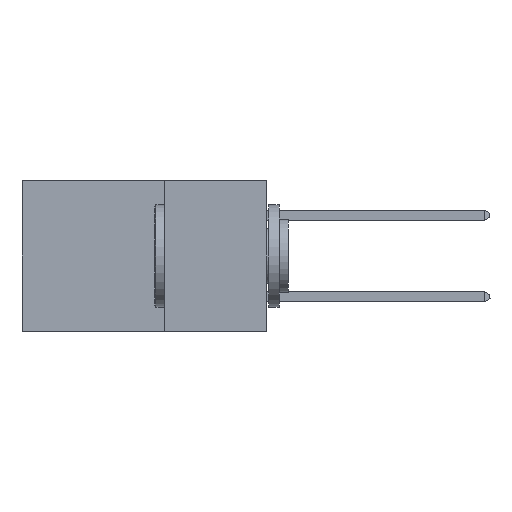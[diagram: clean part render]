
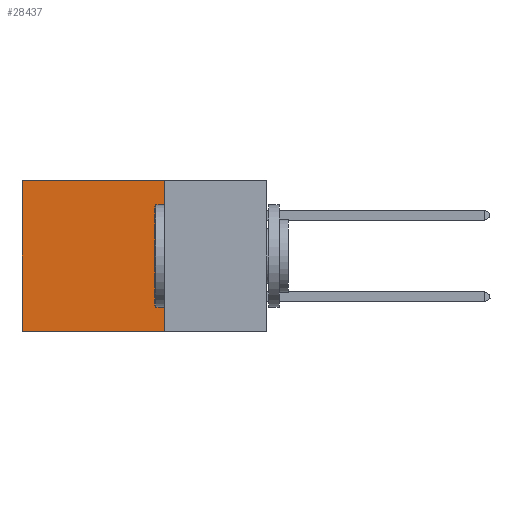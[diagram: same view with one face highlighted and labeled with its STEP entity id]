
A CAD part, left-side view. The second image highlights one B-rep face of the part: STEP entity #28437.
In plain terms, the highlighted planar face has unit normal (-1, 0, 0).
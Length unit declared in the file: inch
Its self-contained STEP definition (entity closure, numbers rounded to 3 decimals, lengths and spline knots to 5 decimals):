
#145 = CARTESIAN_POINT ( 'NONE',  ( 0.2875, 0.25, 0. ) ) ;
#192 = DIRECTION ( 'NONE',  ( 0., 1., 0. ) ) ;
#413 = CARTESIAN_POINT ( 'NONE',  ( 0.2875, 0.25, -0.37 ) ) ;
#705 = VERTEX_POINT ( 'NONE', #12265 ) ;
#2014 = VECTOR ( 'NONE', #17488, 39.37008 ) ;
#2131 = EDGE_CURVE ( 'NONE', #24202, #2950, #23606, .T. ) ;
#2950 = VERTEX_POINT ( 'NONE', #413 ) ;
#4762 = CARTESIAN_POINT ( 'NONE',  ( 0.2875, 0.25, -0.37 ) ) ;
#5652 = VECTOR ( 'NONE', #17753, 39.37008 ) ;
#5959 = EDGE_LOOP ( 'NONE', ( #19941, #28131, #9766, #14712 ) ) ;
#6461 = CARTESIAN_POINT ( 'NONE',  ( 0.2875, 0.6, -0.37 ) ) ;
#6471 = CARTESIAN_POINT ( 'NONE',  ( 0.2875, 0.25, 0. ) ) ;
#7491 = DIRECTION ( 'NONE',  ( 1., 0., 0. ) ) ;
#9766 = ORIENTED_EDGE ( 'NONE', *, *, #2131, .F. ) ;
#10744 = CARTESIAN_POINT ( 'NONE',  ( 0.2875, 0.6, 0. ) ) ;
#11855 = CARTESIAN_POINT ( 'NONE',  ( 0.2875, 0.25, 0. ) ) ;
#11908 = LINE ( 'NONE', #4762, #23096 ) ;
#12038 = CARTESIAN_POINT ( 'NONE',  ( 0.2875, 0.25, 0. ) ) ;
#12058 = EDGE_CURVE ( 'NONE', #2950, #16586, #11908, .T. ) ;
#12265 = CARTESIAN_POINT ( 'NONE',  ( 0.2875, 0.6, 0. ) ) ;
#14124 = DIRECTION ( 'NONE',  ( 0., 1., 0. ) ) ;
#14340 = VECTOR ( 'NONE', #14124, 39.37008 ) ;
#14712 = ORIENTED_EDGE ( 'NONE', *, *, #19378, .T. ) ;
#14802 = LINE ( 'NONE', #10744, #2014 ) ;
#15513 = FACE_OUTER_BOUND ( 'NONE', #5959, .T. ) ;
#16586 = VERTEX_POINT ( 'NONE', #6461 ) ;
#17488 = DIRECTION ( 'NONE',  ( 0., 0., -1. ) ) ;
#17753 = DIRECTION ( 'NONE',  ( 0., 0., -1. ) ) ;
#19378 = EDGE_CURVE ( 'NONE', #24202, #705, #26209, .T. ) ;
#19941 = ORIENTED_EDGE ( 'NONE', *, *, #22811, .T. ) ;
#21040 = PLANE ( 'NONE',  #24646 ) ;
#22811 = EDGE_CURVE ( 'NONE', #705, #16586, #14802, .T. ) ;
#23096 = VECTOR ( 'NONE', #192, 39.37008 ) ;
#23277 = DIRECTION ( 'NONE',  ( 0., 0., -1. ) ) ;
#23606 = LINE ( 'NONE', #6471, #5652 ) ;
#24202 = VERTEX_POINT ( 'NONE', #145 ) ;
#24646 = AXIS2_PLACEMENT_3D ( 'NONE', #12038, #7491, #23277 ) ;
#26209 = LINE ( 'NONE', #11855, #14340 ) ;
#28131 = ORIENTED_EDGE ( 'NONE', *, *, #12058, .F. ) ;
#28437 = ADVANCED_FACE ( 'NONE', ( #15513 ), #21040, .F. ) ;
